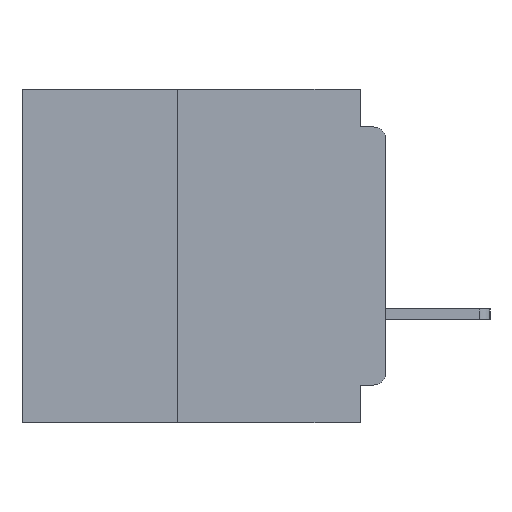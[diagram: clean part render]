
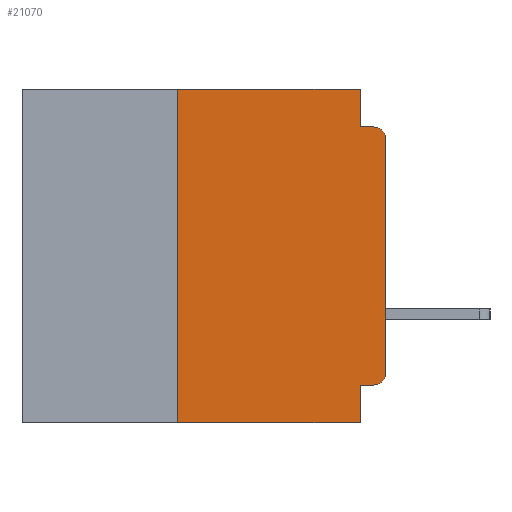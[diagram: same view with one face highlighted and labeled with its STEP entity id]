
A CAD part, left-side view. The second image highlights one B-rep face of the part: STEP entity #21070.
In plain terms, the highlighted planar face has unit normal (-1, 0, 0).
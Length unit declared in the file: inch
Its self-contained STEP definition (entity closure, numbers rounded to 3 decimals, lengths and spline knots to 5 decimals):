
#261 = VERTEX_POINT ( 'NONE', #1639 ) ;
#430 = VERTEX_POINT ( 'NONE', #27449 ) ;
#1032 = CARTESIAN_POINT ( 'NONE',  ( 0., 0.015, -0.045 ) ) ;
#1639 = CARTESIAN_POINT ( 'NONE',  ( 0., 0.25, 0. ) ) ;
#1931 = CARTESIAN_POINT ( 'NONE',  ( 0., 0.437, 0. ) ) ;
#2043 = DIRECTION ( 'NONE',  ( 0., 0., -1. ) ) ;
#3629 = AXIS2_PLACEMENT_3D ( 'NONE', #35013, #13320, #38599 ) ;
#4683 = VECTOR ( 'NONE', #2043, 39.37008 ) ;
#5415 = DIRECTION ( 'NONE',  ( 1., 0., 0. ) ) ;
#5558 = PLANE ( 'NONE',  #8572 ) ;
#5730 = VERTEX_POINT ( 'NONE', #14514 ) ;
#5866 = LINE ( 'NONE', #10598, #34791 ) ;
#6043 = CARTESIAN_POINT ( 'NONE',  ( 0., 0.437, -0.4 ) ) ;
#6053 = ORIENTED_EDGE ( 'NONE', *, *, #40317, .F. ) ;
#6269 = LINE ( 'NONE', #23079, #44676 ) ;
#6350 = LINE ( 'NONE', #39705, #25712 ) ;
#6967 = EDGE_CURVE ( 'NONE', #31650, #39944, #6269, .T. ) ;
#7814 = VECTOR ( 'NONE', #28418, 39.37008 ) ;
#8572 = AXIS2_PLACEMENT_3D ( 'NONE', #1931, #5415, #9201 ) ;
#8831 = EDGE_CURVE ( 'NONE', #35617, #25691, #46131, .T. ) ;
#9201 = DIRECTION ( 'NONE',  ( 0., 0., -1. ) ) ;
#10598 = CARTESIAN_POINT ( 'NONE',  ( 0., 0.031, -0.4 ) ) ;
#10936 = DIRECTION ( 'NONE',  ( 0., -1., 0. ) ) ;
#11056 = LINE ( 'NONE', #14582, #38737 ) ;
#13320 = DIRECTION ( 'NONE',  ( -1., 0., 0. ) ) ;
#13432 = ORIENTED_EDGE ( 'NONE', *, *, #13868, .T. ) ;
#13535 = EDGE_CURVE ( 'NONE', #39944, #29253, #21385, .T. ) ;
#13868 = EDGE_CURVE ( 'NONE', #430, #45307, #25940, .T. ) ;
#14514 = CARTESIAN_POINT ( 'NONE',  ( 0., 0.031, -0.045 ) ) ;
#14582 = CARTESIAN_POINT ( 'NONE',  ( 0., 0., -0.045 ) ) ;
#14610 = EDGE_CURVE ( 'NONE', #5730, #29253, #11056, .T. ) ;
#14876 = CARTESIAN_POINT ( 'NONE',  ( 0., 0.437, 0. ) ) ;
#14886 = CIRCLE ( 'NONE', #3629, 0.015 ) ;
#15005 = DIRECTION ( 'NONE',  ( -1., 0., 0. ) ) ;
#18641 = EDGE_CURVE ( 'NONE', #35617, #31650, #14886, .T. ) ;
#19107 = CARTESIAN_POINT ( 'NONE',  ( 0., 0.031, -0.355 ) ) ;
#19790 = FACE_OUTER_BOUND ( 'NONE', #25668, .T. ) ;
#19856 = CARTESIAN_POINT ( 'NONE',  ( 0., 0., -0.34 ) ) ;
#20111 = CARTESIAN_POINT ( 'NONE',  ( 0., 0.031, 0. ) ) ;
#21070 = ADVANCED_FACE ( 'NONE', ( #19790 ), #5558, .F. ) ;
#21385 = CIRCLE ( 'NONE', #46649, 0.015 ) ;
#21766 = DIRECTION ( 'NONE',  ( 0., 0., 1. ) ) ;
#22087 = CARTESIAN_POINT ( 'NONE',  ( 0., 0., -0.06 ) ) ;
#23079 = CARTESIAN_POINT ( 'NONE',  ( 0., 0., 0. ) ) ;
#23634 = DIRECTION ( 'NONE',  ( 0., 0., 1. ) ) ;
#25319 = ORIENTED_EDGE ( 'NONE', *, *, #6967, .T. ) ;
#25668 = EDGE_LOOP ( 'NONE', ( #25319, #38223, #32109, #28775, #42735, #44989, #13432, #6053, #44479, #41148 ) ) ;
#25691 = VERTEX_POINT ( 'NONE', #19107 ) ;
#25712 = VECTOR ( 'NONE', #21766, 39.37008 ) ;
#25940 = LINE ( 'NONE', #6043, #33271 ) ;
#27449 = CARTESIAN_POINT ( 'NONE',  ( 0., 0.25, -0.4 ) ) ;
#27843 = DIRECTION ( 'NONE',  ( 0., -1., 0. ) ) ;
#28063 = CARTESIAN_POINT ( 'NONE',  ( 0., 0., -0.355 ) ) ;
#28418 = DIRECTION ( 'NONE',  ( 0., 1., 0. ) ) ;
#28575 = EDGE_CURVE ( 'NONE', #261, #38849, #33946, .T. ) ;
#28775 = ORIENTED_EDGE ( 'NONE', *, *, #41179, .F. ) ;
#29253 = VERTEX_POINT ( 'NONE', #1032 ) ;
#29637 = DIRECTION ( 'NONE',  ( 0., -1., 0. ) ) ;
#30104 = CARTESIAN_POINT ( 'NONE',  ( 0., 0.031, 0. ) ) ;
#31650 = VERTEX_POINT ( 'NONE', #19856 ) ;
#32109 = ORIENTED_EDGE ( 'NONE', *, *, #14610, .F. ) ;
#33271 = VECTOR ( 'NONE', #27843, 39.37008 ) ;
#33608 = LINE ( 'NONE', #20111, #4683 ) ;
#33946 = LINE ( 'NONE', #14876, #43409 ) ;
#34120 = CARTESIAN_POINT ( 'NONE',  ( 0., 0.015, -0.355 ) ) ;
#34791 = VECTOR ( 'NONE', #35925, 39.37008 ) ;
#35013 = CARTESIAN_POINT ( 'NONE',  ( 0., 0.015, -0.34 ) ) ;
#35617 = VERTEX_POINT ( 'NONE', #34120 ) ;
#35925 = DIRECTION ( 'NONE',  ( 0., 0., -1. ) ) ;
#36664 = CARTESIAN_POINT ( 'NONE',  ( 0., 0.015, -0.06 ) ) ;
#37690 = EDGE_CURVE ( 'NONE', #430, #261, #6350, .T. ) ;
#38223 = ORIENTED_EDGE ( 'NONE', *, *, #13535, .T. ) ;
#38599 = DIRECTION ( 'NONE',  ( 0., 0., -1. ) ) ;
#38737 = VECTOR ( 'NONE', #10936, 39.37008 ) ;
#38849 = VERTEX_POINT ( 'NONE', #30104 ) ;
#39705 = CARTESIAN_POINT ( 'NONE',  ( 0., 0.25, -0.4 ) ) ;
#39944 = VERTEX_POINT ( 'NONE', #22087 ) ;
#40244 = DIRECTION ( 'NONE',  ( 0., 0., -1. ) ) ;
#40317 = EDGE_CURVE ( 'NONE', #25691, #45307, #5866, .T. ) ;
#41148 = ORIENTED_EDGE ( 'NONE', *, *, #18641, .T. ) ;
#41179 = EDGE_CURVE ( 'NONE', #38849, #5730, #33608, .T. ) ;
#42735 = ORIENTED_EDGE ( 'NONE', *, *, #28575, .F. ) ;
#43409 = VECTOR ( 'NONE', #29637, 39.37008 ) ;
#44479 = ORIENTED_EDGE ( 'NONE', *, *, #8831, .F. ) ;
#44676 = VECTOR ( 'NONE', #23634, 39.37008 ) ;
#44989 = ORIENTED_EDGE ( 'NONE', *, *, #37690, .F. ) ;
#45307 = VERTEX_POINT ( 'NONE', #46002 ) ;
#46002 = CARTESIAN_POINT ( 'NONE',  ( 0., 0.031, -0.4 ) ) ;
#46131 = LINE ( 'NONE', #28063, #7814 ) ;
#46649 = AXIS2_PLACEMENT_3D ( 'NONE', #36664, #15005, #40244 ) ;
